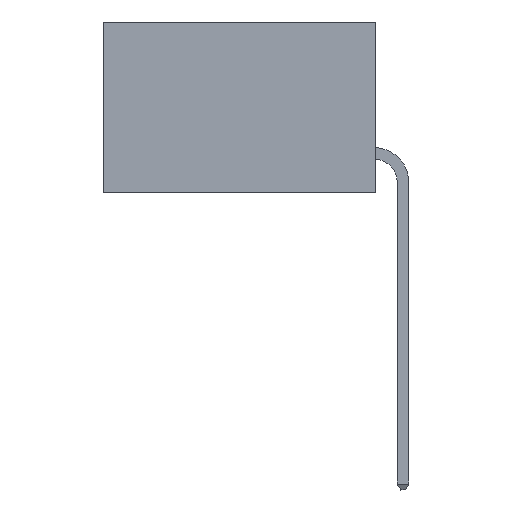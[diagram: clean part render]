
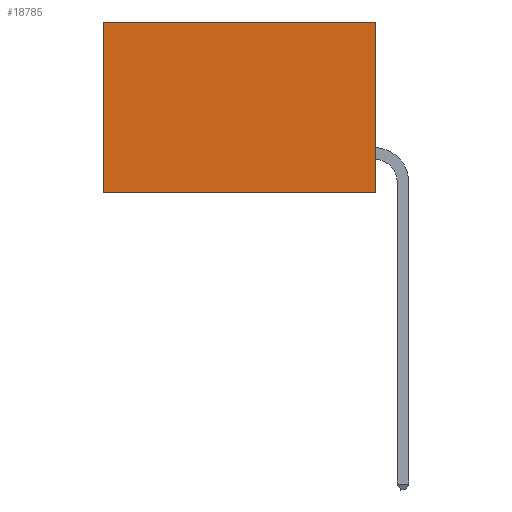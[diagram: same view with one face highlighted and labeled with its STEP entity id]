
A CAD part, left-side view. The second image highlights one B-rep face of the part: STEP entity #18785.
In plain terms, the highlighted planar face has unit normal (-1, 0, 0).
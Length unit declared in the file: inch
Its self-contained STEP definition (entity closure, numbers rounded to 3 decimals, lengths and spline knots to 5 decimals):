
#1280 = PLANE ( 'NONE',  #12791 ) ;
#1966 = ORIENTED_EDGE ( 'NONE', *, *, #22055, .T. ) ;
#3074 = VECTOR ( 'NONE', #10702, 39.37008 ) ;
#3144 = DIRECTION ( 'NONE',  ( 0., 1., 0. ) ) ;
#3200 = VECTOR ( 'NONE', #3144, 39.37008 ) ;
#3452 = DIRECTION ( 'NONE',  ( 0., 0., -1. ) ) ;
#3769 = DIRECTION ( 'NONE',  ( 0., 0., -1. ) ) ;
#6767 = VERTEX_POINT ( 'NONE', #22774 ) ;
#7316 = DIRECTION ( 'NONE',  ( 0., 1., 0. ) ) ;
#8166 = CARTESIAN_POINT ( 'NONE',  ( 0.277, 0., -0.37 ) ) ;
#8310 = CARTESIAN_POINT ( 'NONE',  ( 0.277, 0.59, -0.37 ) ) ;
#9578 = VECTOR ( 'NONE', #7316, 39.37008 ) ;
#9730 = CARTESIAN_POINT ( 'NONE',  ( 0.277, 0., -0.37 ) ) ;
#9788 = LINE ( 'NONE', #22678, #3200 ) ;
#10381 = ORIENTED_EDGE ( 'NONE', *, *, #24773, .F. ) ;
#10702 = DIRECTION ( 'NONE',  ( 0., 0., -1. ) ) ;
#10814 = CARTESIAN_POINT ( 'NONE',  ( 0.277, 0., 0. ) ) ;
#10978 = VECTOR ( 'NONE', #3452, 39.37008 ) ;
#11747 = LINE ( 'NONE', #8310, #10978 ) ;
#12791 = AXIS2_PLACEMENT_3D ( 'NONE', #18325, #18533, #3769 ) ;
#13578 = FACE_OUTER_BOUND ( 'NONE', #22912, .T. ) ;
#16890 = LINE ( 'NONE', #9730, #9578 ) ;
#18236 = CARTESIAN_POINT ( 'NONE',  ( 0.277, 0.59, -0.37 ) ) ;
#18325 = CARTESIAN_POINT ( 'NONE',  ( 0.277, 0., -0.37 ) ) ;
#18533 = DIRECTION ( 'NONE',  ( 1., 0., 0. ) ) ;
#18785 = ADVANCED_FACE ( 'NONE', ( #13578 ), #1280, .F. ) ;
#19290 = EDGE_CURVE ( 'NONE', #19371, #26927, #22662, .T. ) ;
#19371 = VERTEX_POINT ( 'NONE', #10814 ) ;
#22055 = EDGE_CURVE ( 'NONE', #6767, #24381, #11747, .T. ) ;
#22585 = ORIENTED_EDGE ( 'NONE', *, *, #19290, .F. ) ;
#22662 = LINE ( 'NONE', #8166, #3074 ) ;
#22678 = CARTESIAN_POINT ( 'NONE',  ( 0.277, 0., 0. ) ) ;
#22774 = CARTESIAN_POINT ( 'NONE',  ( 0.277, 0.59, 0. ) ) ;
#22912 = EDGE_LOOP ( 'NONE', ( #1966, #10381, #22585, #23766 ) ) ;
#23766 = ORIENTED_EDGE ( 'NONE', *, *, #27067, .T. ) ;
#24381 = VERTEX_POINT ( 'NONE', #18236 ) ;
#24773 = EDGE_CURVE ( 'NONE', #26927, #24381, #16890, .T. ) ;
#26927 = VERTEX_POINT ( 'NONE', #29409 ) ;
#27067 = EDGE_CURVE ( 'NONE', #19371, #6767, #9788, .T. ) ;
#29409 = CARTESIAN_POINT ( 'NONE',  ( 0.277, 0., -0.37 ) ) ;
